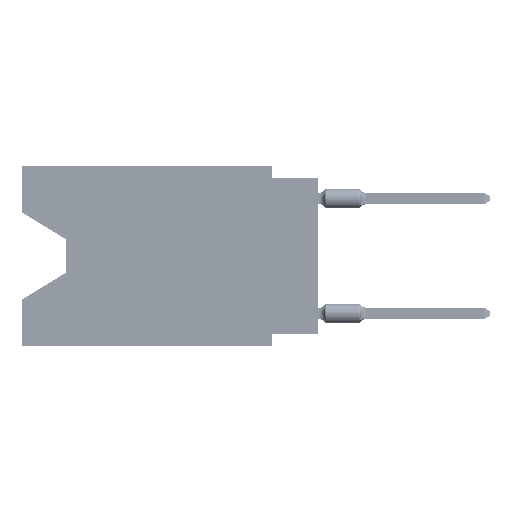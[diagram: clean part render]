
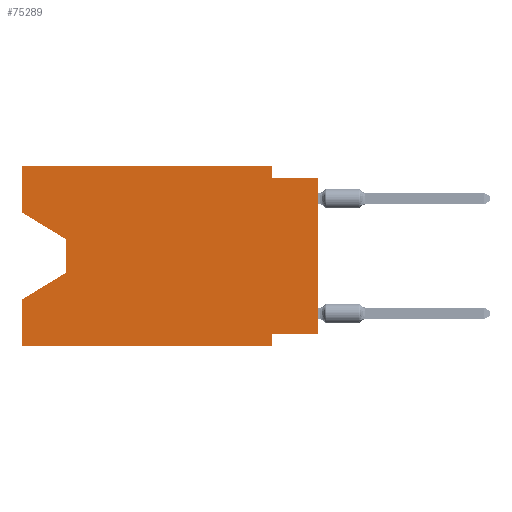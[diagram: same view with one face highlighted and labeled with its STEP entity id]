
A CAD part, left-side view. The second image highlights one B-rep face of the part: STEP entity #75289.
In plain terms, the highlighted planar face has unit normal (-1, 0, 0).
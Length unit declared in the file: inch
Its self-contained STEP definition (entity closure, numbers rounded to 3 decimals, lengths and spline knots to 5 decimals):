
#366 = ORIENTED_EDGE ( 'NONE', *, *, #26197, .T. ) ;
#572 = CARTESIAN_POINT ( 'NONE',  ( 0., 0., -0.365 ) ) ;
#2755 = LINE ( 'NONE', #76260, #20017 ) ;
#2907 = CARTESIAN_POINT ( 'NONE',  ( 0., 0.645, 0. ) ) ;
#3272 = EDGE_CURVE ( 'NONE', #64800, #49081, #56237, .T. ) ;
#5439 = CARTESIAN_POINT ( 'NONE',  ( 0., 0., 0. ) ) ;
#6361 = VERTEX_POINT ( 'NONE', #27401 ) ;
#6979 = VERTEX_POINT ( 'NONE', #7632 ) ;
#7632 = CARTESIAN_POINT ( 'NONE',  ( 0., 0., -0.025 ) ) ;
#7696 = LINE ( 'NONE', #38162, #35806 ) ;
#8125 = VERTEX_POINT ( 'NONE', #56026 ) ;
#9019 = DIRECTION ( 'NONE',  ( 0., 0., 1. ) ) ;
#9688 = LINE ( 'NONE', #69807, #73934 ) ;
#9992 = CARTESIAN_POINT ( 'NONE',  ( 0., 0.645, -0.28975 ) ) ;
#10320 = ORIENTED_EDGE ( 'NONE', *, *, #70976, .F. ) ;
#10688 = CARTESIAN_POINT ( 'NONE',  ( 0., 0., -0.365 ) ) ;
#11214 = LINE ( 'NONE', #35973, #50075 ) ;
#11518 = CARTESIAN_POINT ( 'NONE',  ( 0., 0.1, -0.39 ) ) ;
#11799 = EDGE_CURVE ( 'NONE', #49081, #76528, #22071, .T. ) ;
#13191 = EDGE_CURVE ( 'NONE', #65544, #6979, #66240, .T. ) ;
#13267 = VECTOR ( 'NONE', #26269, 39.37008 ) ;
#13990 = EDGE_CURVE ( 'NONE', #45005, #6361, #77815, .T. ) ;
#15897 = CARTESIAN_POINT ( 'NONE',  ( 0., 0., -0.025 ) ) ;
#18266 = ORIENTED_EDGE ( 'NONE', *, *, #24329, .F. ) ;
#18365 = DIRECTION ( 'NONE',  ( 0., 0., -1. ) ) ;
#18614 = ORIENTED_EDGE ( 'NONE', *, *, #13990, .T. ) ;
#19149 = DIRECTION ( 'NONE',  ( 0., -1., 0. ) ) ;
#19242 = VECTOR ( 'NONE', #32659, 39.37008 ) ;
#20017 = VECTOR ( 'NONE', #33237, 39.37008 ) ;
#20095 = CARTESIAN_POINT ( 'NONE',  ( 0., 0.645, -0.10025 ) ) ;
#20539 = VERTEX_POINT ( 'NONE', #9992 ) ;
#22002 = CARTESIAN_POINT ( 'NONE',  ( 0., 0.1, -0.365 ) ) ;
#22071 = LINE ( 'NONE', #11518, #33261 ) ;
#22385 = DIRECTION ( 'NONE',  ( 0., -1., 0. ) ) ;
#22923 = VECTOR ( 'NONE', #31009, 39.37008 ) ;
#23736 = ORIENTED_EDGE ( 'NONE', *, *, #33678, .T. ) ;
#24329 = EDGE_CURVE ( 'NONE', #77471, #68350, #7696, .T. ) ;
#24483 = CARTESIAN_POINT ( 'NONE',  ( 0., 0.1, -0.39 ) ) ;
#26197 = EDGE_CURVE ( 'NONE', #6361, #20539, #11214, .T. ) ;
#26269 = DIRECTION ( 'NONE',  ( 0., 0., -1. ) ) ;
#26763 = CARTESIAN_POINT ( 'NONE',  ( 0., 0.1, -0.025 ) ) ;
#27401 = CARTESIAN_POINT ( 'NONE',  ( 0., 0.55, -0.232 ) ) ;
#31009 = DIRECTION ( 'NONE',  ( 0., 0., 1. ) ) ;
#31427 = ORIENTED_EDGE ( 'NONE', *, *, #42163, .F. ) ;
#31487 = DIRECTION ( 'NONE',  ( 0., 0.855, -0.519 ) ) ;
#32296 = VECTOR ( 'NONE', #35587, 39.37008 ) ;
#32465 = DIRECTION ( 'NONE',  ( 0., 0., 1. ) ) ;
#32659 = DIRECTION ( 'NONE',  ( 0., 1., 0. ) ) ;
#33237 = DIRECTION ( 'NONE',  ( 0., -0.855, -0.519 ) ) ;
#33261 = VECTOR ( 'NONE', #72816, 39.37008 ) ;
#33357 = CARTESIAN_POINT ( 'NONE',  ( 0., 0.55, -0.158 ) ) ;
#33678 = EDGE_CURVE ( 'NONE', #8125, #76528, #9688, .T. ) ;
#34954 = ORIENTED_EDGE ( 'NONE', *, *, #3272, .F. ) ;
#35587 = DIRECTION ( 'NONE',  ( 0., 0., -1. ) ) ;
#35806 = VECTOR ( 'NONE', #32465, 39.37008 ) ;
#35973 = CARTESIAN_POINT ( 'NONE',  ( 0., 0.55, -0.232 ) ) ;
#37864 = CARTESIAN_POINT ( 'NONE',  ( 0., 0.645, 0. ) ) ;
#38162 = CARTESIAN_POINT ( 'NONE',  ( 0., 0.645, 0. ) ) ;
#38455 = LINE ( 'NONE', #63211, #13267 ) ;
#38887 = AXIS2_PLACEMENT_3D ( 'NONE', #37864, #62229, #18365 ) ;
#38954 = DIRECTION ( 'NONE',  ( 0., -1., 0. ) ) ;
#40519 = EDGE_CURVE ( 'NONE', #77471, #45005, #2755, .T. ) ;
#41089 = LINE ( 'NONE', #2907, #55966 ) ;
#41423 = CARTESIAN_POINT ( 'NONE',  ( 0., 0.645, 0. ) ) ;
#42163 = EDGE_CURVE ( 'NONE', #45606, #65544, #38455, .T. ) ;
#45005 = VERTEX_POINT ( 'NONE', #33357 ) ;
#45606 = VERTEX_POINT ( 'NONE', #68508 ) ;
#49081 = VERTEX_POINT ( 'NONE', #22002 ) ;
#50075 = VECTOR ( 'NONE', #31487, 39.37008 ) ;
#51594 = VECTOR ( 'NONE', #19149, 39.37008 ) ;
#51849 = ORIENTED_EDGE ( 'NONE', *, *, #11799, .F. ) ;
#53950 = ORIENTED_EDGE ( 'NONE', *, *, #56914, .T. ) ;
#54553 = FACE_OUTER_BOUND ( 'NONE', #64568, .T. ) ;
#55348 = PLANE ( 'NONE',  #38887 ) ;
#55966 = VECTOR ( 'NONE', #9019, 39.37008 ) ;
#56026 = CARTESIAN_POINT ( 'NONE',  ( 0., 0.645, -0.39 ) ) ;
#56237 = LINE ( 'NONE', #572, #19242 ) ;
#56310 = ORIENTED_EDGE ( 'NONE', *, *, #40519, .T. ) ;
#56914 = EDGE_CURVE ( 'NONE', #64800, #6979, #61070, .T. ) ;
#61070 = LINE ( 'NONE', #5439, #22923 ) ;
#62229 = DIRECTION ( 'NONE',  ( 1., 0., 0. ) ) ;
#62609 = CARTESIAN_POINT ( 'NONE',  ( 0., 0.645, 0. ) ) ;
#63211 = CARTESIAN_POINT ( 'NONE',  ( 0., 0.1, 0. ) ) ;
#63945 = ORIENTED_EDGE ( 'NONE', *, *, #13191, .F. ) ;
#64568 = EDGE_LOOP ( 'NONE', ( #56310, #18614, #366, #73655, #23736, #51849, #34954, #53950, #63945, #31427, #10320, #18266 ) ) ;
#64800 = VERTEX_POINT ( 'NONE', #10688 ) ;
#65544 = VERTEX_POINT ( 'NONE', #26763 ) ;
#66240 = LINE ( 'NONE', #15897, #75980 ) ;
#68350 = VERTEX_POINT ( 'NONE', #41423 ) ;
#68508 = CARTESIAN_POINT ( 'NONE',  ( 0., 0.1, 0. ) ) ;
#69807 = CARTESIAN_POINT ( 'NONE',  ( 0., 0.645, -0.39 ) ) ;
#70976 = EDGE_CURVE ( 'NONE', #68350, #45606, #74776, .T. ) ;
#71735 = CARTESIAN_POINT ( 'NONE',  ( 0., 0.55, -0.158 ) ) ;
#72816 = DIRECTION ( 'NONE',  ( 0., 0., -1. ) ) ;
#73655 = ORIENTED_EDGE ( 'NONE', *, *, #79603, .F. ) ;
#73934 = VECTOR ( 'NONE', #38954, 39.37008 ) ;
#74776 = LINE ( 'NONE', #62609, #51594 ) ;
#75289 = ADVANCED_FACE ( 'NONE', ( #54553 ), #55348, .F. ) ;
#75980 = VECTOR ( 'NONE', #22385, 39.37008 ) ;
#76260 = CARTESIAN_POINT ( 'NONE',  ( 0., 0.645, -0.10025 ) ) ;
#76528 = VERTEX_POINT ( 'NONE', #24483 ) ;
#77471 = VERTEX_POINT ( 'NONE', #20095 ) ;
#77815 = LINE ( 'NONE', #71735, #32296 ) ;
#79603 = EDGE_CURVE ( 'NONE', #8125, #20539, #41089, .T. ) ;
